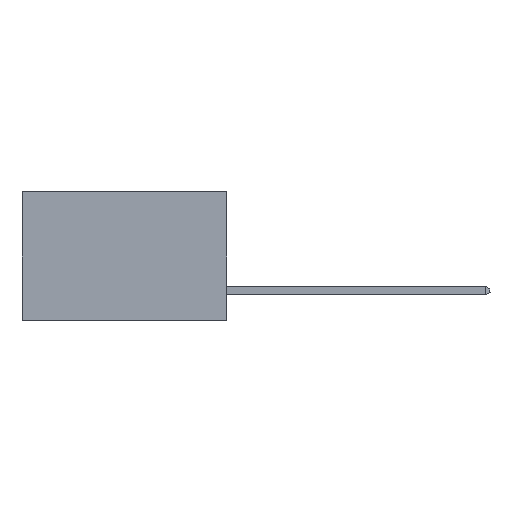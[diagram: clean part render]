
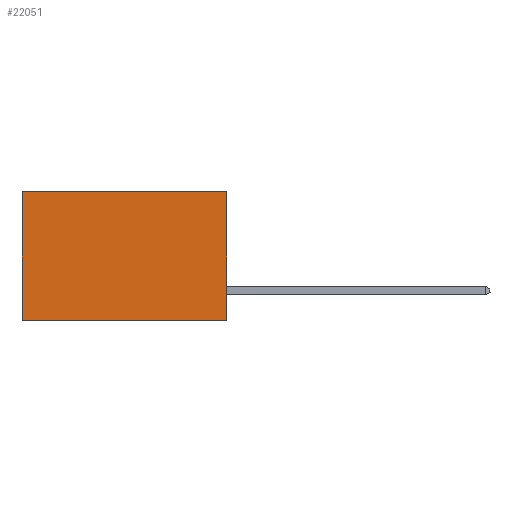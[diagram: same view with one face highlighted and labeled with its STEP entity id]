
A CAD part, left-side view. The second image highlights one B-rep face of the part: STEP entity #22051.
In plain terms, the highlighted planar face has unit normal (-1, 0, 0).
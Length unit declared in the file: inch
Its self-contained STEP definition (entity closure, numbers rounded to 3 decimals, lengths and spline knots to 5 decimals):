
#178 = DIRECTION ( 'NONE',  ( 0., 0., -1. ) ) ;
#524 = DIRECTION ( 'NONE',  ( 0., 1., 0. ) ) ;
#551 = CARTESIAN_POINT ( 'NONE',  ( 0.277, 0., -0.37 ) ) ;
#649 = ORIENTED_EDGE ( 'NONE', *, *, #18145, .F. ) ;
#1904 = ORIENTED_EDGE ( 'NONE', *, *, #15249, .T. ) ;
#3445 = VECTOR ( 'NONE', #16724, 39.37008 ) ;
#3660 = CARTESIAN_POINT ( 'NONE',  ( 0.277, 0.59, -0.37 ) ) ;
#5359 = LINE ( 'NONE', #12737, #25689 ) ;
#5541 = VERTEX_POINT ( 'NONE', #15218 ) ;
#6296 = DIRECTION ( 'NONE',  ( 0., 1., 0. ) ) ;
#6414 = EDGE_CURVE ( 'NONE', #12268, #13752, #11892, .T. ) ;
#6797 = CARTESIAN_POINT ( 'NONE',  ( 0.277, 0., -0.37 ) ) ;
#7567 = ORIENTED_EDGE ( 'NONE', *, *, #21134, .T. ) ;
#8092 = FACE_OUTER_BOUND ( 'NONE', #16321, .T. ) ;
#9000 = DIRECTION ( 'NONE',  ( 0., 0., -1. ) ) ;
#10843 = VECTOR ( 'NONE', #524, 39.37008 ) ;
#11892 = LINE ( 'NONE', #551, #17676 ) ;
#12268 = VERTEX_POINT ( 'NONE', #17444 ) ;
#12737 = CARTESIAN_POINT ( 'NONE',  ( 0.277, 0., 0. ) ) ;
#13752 = VERTEX_POINT ( 'NONE', #24452 ) ;
#14379 = LINE ( 'NONE', #3660, #3445 ) ;
#15218 = CARTESIAN_POINT ( 'NONE',  ( 0.277, 0.59, -0.37 ) ) ;
#15249 = EDGE_CURVE ( 'NONE', #12268, #21036, #5359, .T. ) ;
#15807 = CARTESIAN_POINT ( 'NONE',  ( 0.277, 0., -0.37 ) ) ;
#16321 = EDGE_LOOP ( 'NONE', ( #7567, #649, #26344, #1904 ) ) ;
#16435 = CARTESIAN_POINT ( 'NONE',  ( 0.277, 0.59, 0. ) ) ;
#16724 = DIRECTION ( 'NONE',  ( 0., 0., -1. ) ) ;
#17444 = CARTESIAN_POINT ( 'NONE',  ( 0.277, 0., 0. ) ) ;
#17676 = VECTOR ( 'NONE', #178, 39.37008 ) ;
#18145 = EDGE_CURVE ( 'NONE', #13752, #5541, #28097, .T. ) ;
#19792 = PLANE ( 'NONE',  #23931 ) ;
#21036 = VERTEX_POINT ( 'NONE', #16435 ) ;
#21134 = EDGE_CURVE ( 'NONE', #21036, #5541, #14379, .T. ) ;
#21938 = DIRECTION ( 'NONE',  ( 1., 0., 0. ) ) ;
#22051 = ADVANCED_FACE ( 'NONE', ( #8092 ), #19792, .F. ) ;
#23931 = AXIS2_PLACEMENT_3D ( 'NONE', #6797, #21938, #9000 ) ;
#24452 = CARTESIAN_POINT ( 'NONE',  ( 0.277, 0., -0.37 ) ) ;
#25689 = VECTOR ( 'NONE', #6296, 39.37008 ) ;
#26344 = ORIENTED_EDGE ( 'NONE', *, *, #6414, .F. ) ;
#28097 = LINE ( 'NONE', #15807, #10843 ) ;
